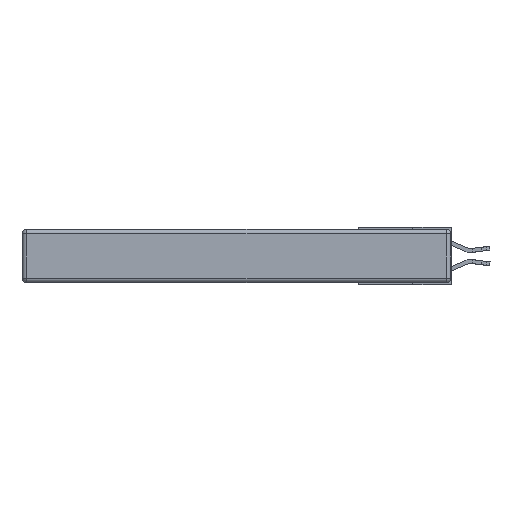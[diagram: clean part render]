
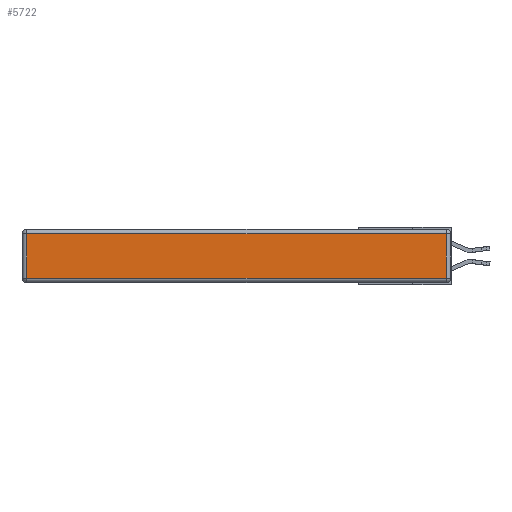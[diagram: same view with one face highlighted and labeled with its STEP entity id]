
A CAD part, left-side view. The second image highlights one B-rep face of the part: STEP entity #5722.
In plain terms, the highlighted planar face has unit normal (-1, 0, 0).
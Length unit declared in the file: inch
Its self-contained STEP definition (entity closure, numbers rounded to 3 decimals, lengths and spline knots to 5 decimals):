
#1520 = LINE ( 'NONE', #3913, #20171 ) ;
#1934 = DIRECTION ( 'NONE',  ( 0., 0., -1. ) ) ;
#2594 = CARTESIAN_POINT ( 'NONE',  ( 0., 0., -0.343 ) ) ;
#2652 = DIRECTION ( 'NONE',  ( 0., 0., 1. ) ) ;
#2868 = VECTOR ( 'NONE', #12742, 39.37008 ) ;
#3562 = EDGE_CURVE ( 'NONE', #8866, #6965, #16684, .T. ) ;
#3913 = CARTESIAN_POINT ( 'NONE',  ( 0., 2.72, -0.343 ) ) ;
#4435 = DIRECTION ( 'NONE',  ( 0., 0., 1. ) ) ;
#4792 = VERTEX_POINT ( 'NONE', #8516 ) ;
#4816 = CARTESIAN_POINT ( 'NONE',  ( 0., 2.72, -0.03 ) ) ;
#4974 = VERTEX_POINT ( 'NONE', #4816 ) ;
#5548 = EDGE_LOOP ( 'NONE', ( #6062, #16183, #16435, #22115 ) ) ;
#5553 = AXIS2_PLACEMENT_3D ( 'NONE', #2594, #15237, #4435 ) ;
#5711 = LINE ( 'NONE', #10853, #2868 ) ;
#5722 = ADVANCED_FACE ( 'NONE', ( #22927 ), #7979, .T. ) ;
#6032 = CARTESIAN_POINT ( 'NONE',  ( 0., 0.03, -0.03 ) ) ;
#6062 = ORIENTED_EDGE ( 'NONE', *, *, #21484, .T. ) ;
#6965 = VERTEX_POINT ( 'NONE', #6032 ) ;
#7979 = PLANE ( 'NONE',  #5553 ) ;
#8516 = CARTESIAN_POINT ( 'NONE',  ( 0., 2.72, -0.313 ) ) ;
#8866 = VERTEX_POINT ( 'NONE', #11142 ) ;
#10260 = EDGE_CURVE ( 'NONE', #4974, #4792, #1520, .T. ) ;
#10853 = CARTESIAN_POINT ( 'NONE',  ( 0., 2.75, -0.03 ) ) ;
#11142 = CARTESIAN_POINT ( 'NONE',  ( 0., 0.03, -0.313 ) ) ;
#12742 = DIRECTION ( 'NONE',  ( 0., 1., 0. ) ) ;
#14777 = CARTESIAN_POINT ( 'NONE',  ( 0., 0., -0.313 ) ) ;
#15237 = DIRECTION ( 'NONE',  ( -1., 0., 0. ) ) ;
#15265 = VECTOR ( 'NONE', #2652, 39.37008 ) ;
#16183 = ORIENTED_EDGE ( 'NONE', *, *, #3562, .T. ) ;
#16435 = ORIENTED_EDGE ( 'NONE', *, *, #17585, .T. ) ;
#16684 = LINE ( 'NONE', #22790, #15265 ) ;
#16755 = VECTOR ( 'NONE', #22064, 39.37008 ) ;
#17585 = EDGE_CURVE ( 'NONE', #6965, #4974, #5711, .T. ) ;
#17599 = LINE ( 'NONE', #14777, #16755 ) ;
#20171 = VECTOR ( 'NONE', #1934, 39.37008 ) ;
#21484 = EDGE_CURVE ( 'NONE', #4792, #8866, #17599, .T. ) ;
#22064 = DIRECTION ( 'NONE',  ( 0., -1., 0. ) ) ;
#22115 = ORIENTED_EDGE ( 'NONE', *, *, #10260, .T. ) ;
#22790 = CARTESIAN_POINT ( 'NONE',  ( 0., 0.03, -0.343 ) ) ;
#22927 = FACE_OUTER_BOUND ( 'NONE', #5548, .T. ) ;
